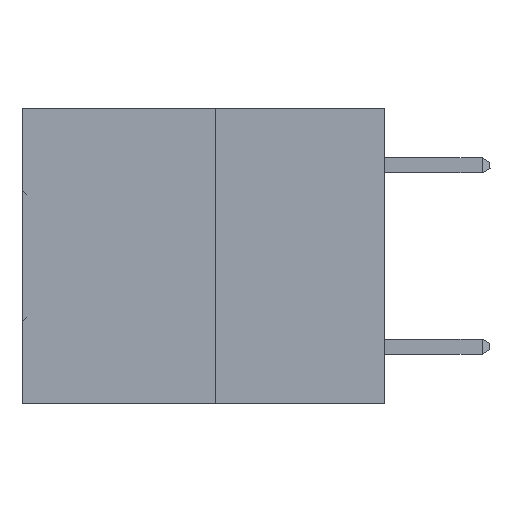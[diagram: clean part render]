
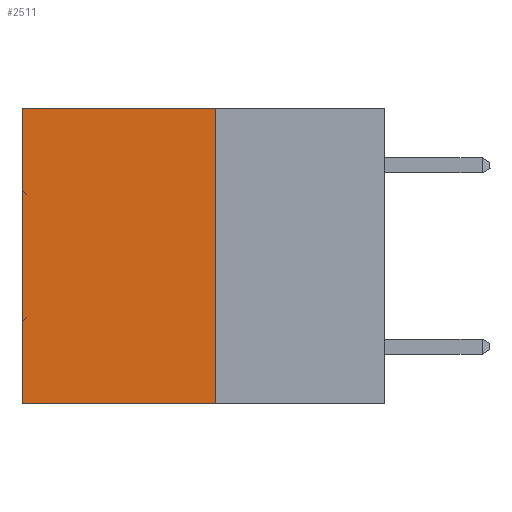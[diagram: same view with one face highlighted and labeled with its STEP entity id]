
A CAD part, left-side view. The second image highlights one B-rep face of the part: STEP entity #2511.
In plain terms, the highlighted planar face has unit normal (-1, 0, 0).
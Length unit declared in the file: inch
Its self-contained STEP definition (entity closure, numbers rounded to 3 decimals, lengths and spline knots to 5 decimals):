
#1905 = CARTESIAN_POINT ( 'NONE',  ( 0.3165, 0.6, 0. ) ) ;
#2254 = ORIENTED_EDGE ( 'NONE', *, *, #25460, .F. ) ;
#2511 = ADVANCED_FACE ( 'NONE', ( #3765 ), #14762, .F. ) ;
#3452 = DIRECTION ( 'NONE',  ( 0., 0., -1. ) ) ;
#3502 = CARTESIAN_POINT ( 'NONE',  ( 0.3165, 0.28, -0.49 ) ) ;
#3765 = FACE_OUTER_BOUND ( 'NONE', #6882, .T. ) ;
#4219 = VECTOR ( 'NONE', #31901, 39.37008 ) ;
#5343 = VERTEX_POINT ( 'NONE', #26882 ) ;
#6882 = EDGE_LOOP ( 'NONE', ( #22915, #2254, #9768, #14016 ) ) ;
#8027 = VERTEX_POINT ( 'NONE', #26735 ) ;
#9768 = ORIENTED_EDGE ( 'NONE', *, *, #28928, .F. ) ;
#11917 = DIRECTION ( 'NONE',  ( 0., 0., -1. ) ) ;
#14016 = ORIENTED_EDGE ( 'NONE', *, *, #36162, .T. ) ;
#14647 = DIRECTION ( 'NONE',  ( 1., 0., 0. ) ) ;
#14762 = PLANE ( 'NONE',  #19867 ) ;
#17283 = CARTESIAN_POINT ( 'NONE',  ( 0.3165, 0.28, 0. ) ) ;
#18668 = VECTOR ( 'NONE', #11917, 39.37008 ) ;
#19867 = AXIS2_PLACEMENT_3D ( 'NONE', #20644, #14647, #3452 ) ;
#20267 = LINE ( 'NONE', #31066, #26040 ) ;
#20644 = CARTESIAN_POINT ( 'NONE',  ( 0.3165, 0.28, -0.49 ) ) ;
#22915 = ORIENTED_EDGE ( 'NONE', *, *, #23691, .T. ) ;
#23369 = CARTESIAN_POINT ( 'NONE',  ( 0.3165, 0.28, -0.49 ) ) ;
#23691 = EDGE_CURVE ( 'NONE', #27770, #8027, #36623, .T. ) ;
#25077 = DIRECTION ( 'NONE',  ( 0., 0., -1. ) ) ;
#25163 = LINE ( 'NONE', #3502, #4219 ) ;
#25203 = DIRECTION ( 'NONE',  ( 0., 1., 0. ) ) ;
#25460 = EDGE_CURVE ( 'NONE', #5343, #8027, #25163, .T. ) ;
#26040 = VECTOR ( 'NONE', #25203, 39.37008 ) ;
#26249 = LINE ( 'NONE', #23369, #18668 ) ;
#26735 = CARTESIAN_POINT ( 'NONE',  ( 0.3165, 0.6, -0.49 ) ) ;
#26882 = CARTESIAN_POINT ( 'NONE',  ( 0.3165, 0.28, -0.49 ) ) ;
#27770 = VERTEX_POINT ( 'NONE', #1905 ) ;
#28928 = EDGE_CURVE ( 'NONE', #33766, #5343, #26249, .T. ) ;
#31066 = CARTESIAN_POINT ( 'NONE',  ( 0.3165, 0.28, 0. ) ) ;
#31901 = DIRECTION ( 'NONE',  ( 0., 1., 0. ) ) ;
#33766 = VERTEX_POINT ( 'NONE', #17283 ) ;
#33899 = VECTOR ( 'NONE', #25077, 39.37008 ) ;
#36051 = CARTESIAN_POINT ( 'NONE',  ( 0.3165, 0.6, -0.49 ) ) ;
#36162 = EDGE_CURVE ( 'NONE', #33766, #27770, #20267, .T. ) ;
#36623 = LINE ( 'NONE', #36051, #33899 ) ;
